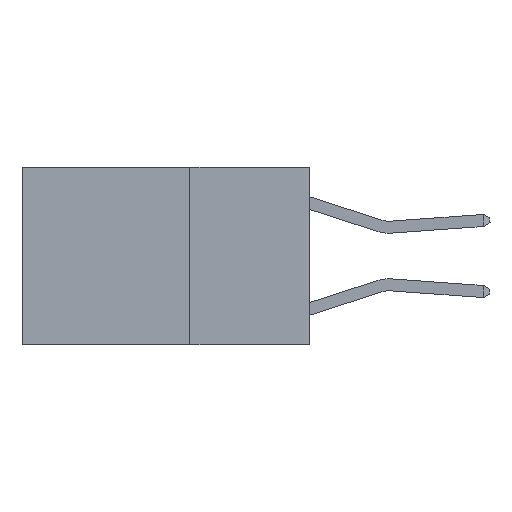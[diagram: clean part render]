
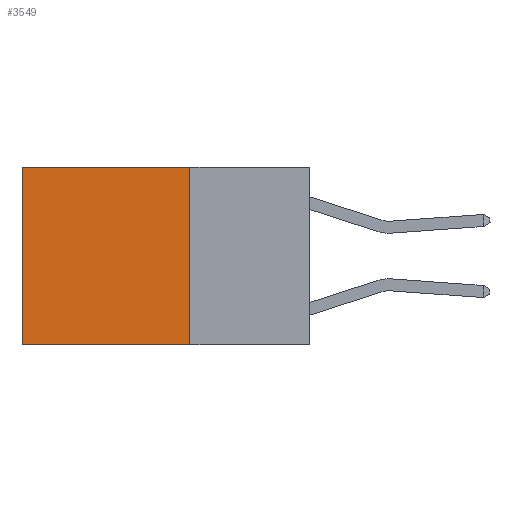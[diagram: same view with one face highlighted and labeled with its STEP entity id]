
A CAD part, left-side view. The second image highlights one B-rep face of the part: STEP entity #3549.
In plain terms, the highlighted planar face has unit normal (-1, 0, 0).
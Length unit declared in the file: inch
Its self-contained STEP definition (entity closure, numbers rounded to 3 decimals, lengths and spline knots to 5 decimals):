
#252 = ORIENTED_EDGE ( 'NONE', *, *, #17861, .T. ) ;
#2362 = VERTEX_POINT ( 'NONE', #10292 ) ;
#2508 = EDGE_CURVE ( 'NONE', #13343, #2362, #13530, .T. ) ;
#2814 = VECTOR ( 'NONE', #13719, 39.37008 ) ;
#3037 = DIRECTION ( 'NONE',  ( 0., 0., -1. ) ) ;
#3074 = PLANE ( 'NONE',  #7810 ) ;
#3549 = ADVANCED_FACE ( 'NONE', ( #7137 ), #3074, .F. ) ;
#4051 = CARTESIAN_POINT ( 'NONE',  ( 0.2625, 0.25, 0. ) ) ;
#4403 = LINE ( 'NONE', #10088, #14969 ) ;
#5128 = VECTOR ( 'NONE', #8708, 39.37008 ) ;
#5550 = LINE ( 'NONE', #7040, #5128 ) ;
#5997 = DIRECTION ( 'NONE',  ( 0., 0., -1. ) ) ;
#6866 = VECTOR ( 'NONE', #12564, 39.37008 ) ;
#7040 = CARTESIAN_POINT ( 'NONE',  ( 0.2625, 0.25, -0.37 ) ) ;
#7066 = CARTESIAN_POINT ( 'NONE',  ( 0.2625, 0.25, 0. ) ) ;
#7137 = FACE_OUTER_BOUND ( 'NONE', #17719, .T. ) ;
#7163 = VERTEX_POINT ( 'NONE', #17164 ) ;
#7310 = LINE ( 'NONE', #7066, #6866 ) ;
#7810 = AXIS2_PLACEMENT_3D ( 'NONE', #12859, #14208, #5997 ) ;
#8708 = DIRECTION ( 'NONE',  ( 0., 1., 0. ) ) ;
#9194 = CARTESIAN_POINT ( 'NONE',  ( 0.2625, 0.6, -0.37 ) ) ;
#10088 = CARTESIAN_POINT ( 'NONE',  ( 0.2625, 0.6, 0. ) ) ;
#10292 = CARTESIAN_POINT ( 'NONE',  ( 0.2625, 0.25, -0.37 ) ) ;
#10403 = ORIENTED_EDGE ( 'NONE', *, *, #10525, .T. ) ;
#10525 = EDGE_CURVE ( 'NONE', #7163, #16540, #4403, .T. ) ;
#10825 = ORIENTED_EDGE ( 'NONE', *, *, #16229, .F. ) ;
#12564 = DIRECTION ( 'NONE',  ( 0., 1., 0. ) ) ;
#12859 = CARTESIAN_POINT ( 'NONE',  ( 0.2625, 0.25, 0. ) ) ;
#13343 = VERTEX_POINT ( 'NONE', #16309 ) ;
#13530 = LINE ( 'NONE', #4051, #2814 ) ;
#13719 = DIRECTION ( 'NONE',  ( 0., 0., -1. ) ) ;
#14208 = DIRECTION ( 'NONE',  ( 1., 0., 0. ) ) ;
#14448 = ORIENTED_EDGE ( 'NONE', *, *, #2508, .F. ) ;
#14969 = VECTOR ( 'NONE', #3037, 39.37008 ) ;
#16229 = EDGE_CURVE ( 'NONE', #2362, #16540, #5550, .T. ) ;
#16309 = CARTESIAN_POINT ( 'NONE',  ( 0.2625, 0.25, 0. ) ) ;
#16540 = VERTEX_POINT ( 'NONE', #9194 ) ;
#17164 = CARTESIAN_POINT ( 'NONE',  ( 0.2625, 0.6, 0. ) ) ;
#17719 = EDGE_LOOP ( 'NONE', ( #10403, #10825, #14448, #252 ) ) ;
#17861 = EDGE_CURVE ( 'NONE', #13343, #7163, #7310, .T. ) ;
